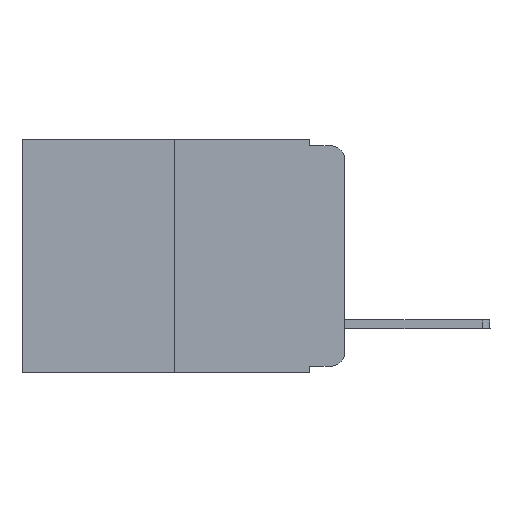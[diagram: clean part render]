
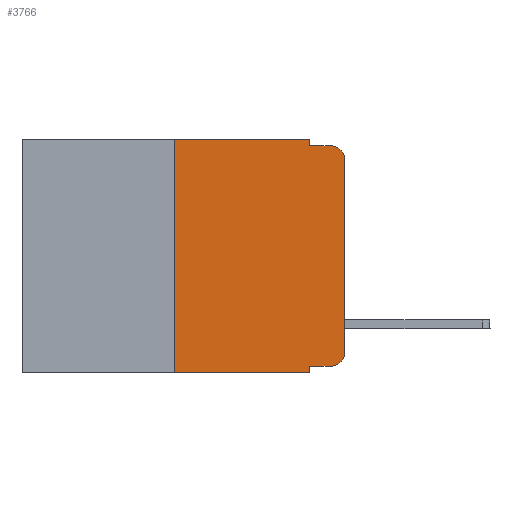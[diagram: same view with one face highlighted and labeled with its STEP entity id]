
A CAD part, left-side view. The second image highlights one B-rep face of the part: STEP entity #3766.
In plain terms, the highlighted planar face has unit normal (-1, 0, 0).
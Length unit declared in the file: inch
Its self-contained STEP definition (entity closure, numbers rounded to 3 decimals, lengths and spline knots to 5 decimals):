
#7 = DIRECTION ( 'NONE',  ( 0., 0., 1. ) ) ;
#176 = CARTESIAN_POINT ( 'NONE',  ( 0., 0.051, 0. ) ) ;
#377 = DIRECTION ( 'NONE',  ( 0., 0., 1. ) ) ;
#416 = EDGE_CURVE ( 'NONE', #12842, #7897, #3787, .T. ) ;
#417 = DIRECTION ( 'NONE',  ( 0., 0., -1. ) ) ;
#515 = ORIENTED_EDGE ( 'NONE', *, *, #1745, .T. ) ;
#1016 = VERTEX_POINT ( 'NONE', #10771 ) ;
#1371 = DIRECTION ( 'NONE',  ( 0., 0., -1. ) ) ;
#1684 = ORIENTED_EDGE ( 'NONE', *, *, #9439, .F. ) ;
#1745 = EDGE_CURVE ( 'NONE', #3607, #1016, #15521, .T. ) ;
#1774 = LINE ( 'NONE', #12016, #13179 ) ;
#2016 = AXIS2_PLACEMENT_3D ( 'NONE', #10759, #4242, #1371 ) ;
#2163 = EDGE_LOOP ( 'NONE', ( #7395, #8749, #16146, #10981, #8238, #12766, #2238, #1684, #12142, #515 ) ) ;
#2238 = ORIENTED_EDGE ( 'NONE', *, *, #416, .T. ) ;
#2339 = VERTEX_POINT ( 'NONE', #3645 ) ;
#2412 = CARTESIAN_POINT ( 'NONE',  ( 0., 0.051, -0.01 ) ) ;
#2448 = CARTESIAN_POINT ( 'NONE',  ( 0., 0.02, -0.333 ) ) ;
#2539 = EDGE_CURVE ( 'NONE', #2339, #11720, #11095, .T. ) ;
#2735 = DIRECTION ( 'NONE',  ( 0., 0., -1. ) ) ;
#3312 = VERTEX_POINT ( 'NONE', #15055 ) ;
#3504 = AXIS2_PLACEMENT_3D ( 'NONE', #8109, #14723, #417 ) ;
#3554 = CARTESIAN_POINT ( 'NONE',  ( 0., 0.051, 0. ) ) ;
#3607 = VERTEX_POINT ( 'NONE', #2448 ) ;
#3645 = CARTESIAN_POINT ( 'NONE',  ( 0., 0.25, 0. ) ) ;
#3766 = ADVANCED_FACE ( 'NONE', ( #5906 ), #15639, .F. ) ;
#3787 = LINE ( 'NONE', #9465, #8649 ) ;
#4175 = LINE ( 'NONE', #13425, #11323 ) ;
#4242 = DIRECTION ( 'NONE',  ( -1., 0., 0. ) ) ;
#4754 = EDGE_CURVE ( 'NONE', #14810, #3607, #7680, .T. ) ;
#5344 = CARTESIAN_POINT ( 'NONE',  ( 0., 0.051, -0.01 ) ) ;
#5352 = VECTOR ( 'NONE', #9296, 39.37008 ) ;
#5906 = FACE_OUTER_BOUND ( 'NONE', #2163, .T. ) ;
#5931 = DIRECTION ( 'NONE',  ( 0., -1., 0. ) ) ;
#6204 = DIRECTION ( 'NONE',  ( 0., 0., -1. ) ) ;
#6216 = CARTESIAN_POINT ( 'NONE',  ( 0., 0.051, -0.333 ) ) ;
#6611 = CARTESIAN_POINT ( 'NONE',  ( 0., 0.25, -0.343 ) ) ;
#6665 = EDGE_CURVE ( 'NONE', #3312, #13804, #13226, .T. ) ;
#7031 = VECTOR ( 'NONE', #6204, 39.37008 ) ;
#7395 = ORIENTED_EDGE ( 'NONE', *, *, #8869, .T. ) ;
#7680 = LINE ( 'NONE', #13692, #13624 ) ;
#7826 = LINE ( 'NONE', #3554, #7031 ) ;
#7897 = VERTEX_POINT ( 'NONE', #9632 ) ;
#8109 = CARTESIAN_POINT ( 'NONE',  ( 0., 0.02, -0.313 ) ) ;
#8238 = ORIENTED_EDGE ( 'NONE', *, *, #2539, .F. ) ;
#8649 = VECTOR ( 'NONE', #9866, 39.37008 ) ;
#8749 = ORIENTED_EDGE ( 'NONE', *, *, #6665, .T. ) ;
#8869 = EDGE_CURVE ( 'NONE', #1016, #3312, #1774, .T. ) ;
#9224 = VERTEX_POINT ( 'NONE', #5344 ) ;
#9296 = DIRECTION ( 'NONE',  ( 0., 0., -1. ) ) ;
#9439 = EDGE_CURVE ( 'NONE', #14810, #7897, #7826, .T. ) ;
#9465 = CARTESIAN_POINT ( 'NONE',  ( 0., 0.473, -0.343 ) ) ;
#9632 = CARTESIAN_POINT ( 'NONE',  ( 0., 0.051, -0.343 ) ) ;
#9866 = DIRECTION ( 'NONE',  ( 0., -1., 0. ) ) ;
#9976 = AXIS2_PLACEMENT_3D ( 'NONE', #11755, #10633, #2735 ) ;
#10491 = LINE ( 'NONE', #2412, #14741 ) ;
#10624 = CARTESIAN_POINT ( 'NONE',  ( 0., 0.473, 0. ) ) ;
#10633 = DIRECTION ( 'NONE',  ( 1., 0., 0. ) ) ;
#10759 = CARTESIAN_POINT ( 'NONE',  ( 0., 0.02, -0.03 ) ) ;
#10771 = CARTESIAN_POINT ( 'NONE',  ( 0., 0., -0.313 ) ) ;
#10960 = EDGE_CURVE ( 'NONE', #11720, #9224, #11289, .T. ) ;
#10981 = ORIENTED_EDGE ( 'NONE', *, *, #10960, .F. ) ;
#11095 = LINE ( 'NONE', #10624, #16325 ) ;
#11289 = LINE ( 'NONE', #176, #5352 ) ;
#11323 = VECTOR ( 'NONE', #377, 39.37008 ) ;
#11720 = VERTEX_POINT ( 'NONE', #15999 ) ;
#11755 = CARTESIAN_POINT ( 'NONE',  ( 0., 0.473, 0. ) ) ;
#11921 = DIRECTION ( 'NONE',  ( 0., -1., 0. ) ) ;
#12016 = CARTESIAN_POINT ( 'NONE',  ( 0., 0., 0. ) ) ;
#12142 = ORIENTED_EDGE ( 'NONE', *, *, #4754, .T. ) ;
#12766 = ORIENTED_EDGE ( 'NONE', *, *, #16309, .F. ) ;
#12842 = VERTEX_POINT ( 'NONE', #6611 ) ;
#13179 = VECTOR ( 'NONE', #7, 39.37008 ) ;
#13226 = CIRCLE ( 'NONE', #2016, 0.02 ) ;
#13425 = CARTESIAN_POINT ( 'NONE',  ( 0., 0.25, 0. ) ) ;
#13538 = CARTESIAN_POINT ( 'NONE',  ( 0., 0.02, -0.01 ) ) ;
#13624 = VECTOR ( 'NONE', #5931, 39.37008 ) ;
#13692 = CARTESIAN_POINT ( 'NONE',  ( 0., 0.051, -0.333 ) ) ;
#13804 = VERTEX_POINT ( 'NONE', #13538 ) ;
#14723 = DIRECTION ( 'NONE',  ( -1., 0., 0. ) ) ;
#14741 = VECTOR ( 'NONE', #15652, 39.37008 ) ;
#14810 = VERTEX_POINT ( 'NONE', #6216 ) ;
#15055 = CARTESIAN_POINT ( 'NONE',  ( 0., 0., -0.03 ) ) ;
#15521 = CIRCLE ( 'NONE', #3504, 0.02 ) ;
#15639 = PLANE ( 'NONE',  #9976 ) ;
#15652 = DIRECTION ( 'NONE',  ( 0., -1., 0. ) ) ;
#15999 = CARTESIAN_POINT ( 'NONE',  ( 0., 0.051, 0. ) ) ;
#16146 = ORIENTED_EDGE ( 'NONE', *, *, #16775, .F. ) ;
#16309 = EDGE_CURVE ( 'NONE', #12842, #2339, #4175, .T. ) ;
#16325 = VECTOR ( 'NONE', #11921, 39.37008 ) ;
#16775 = EDGE_CURVE ( 'NONE', #9224, #13804, #10491, .T. ) ;
